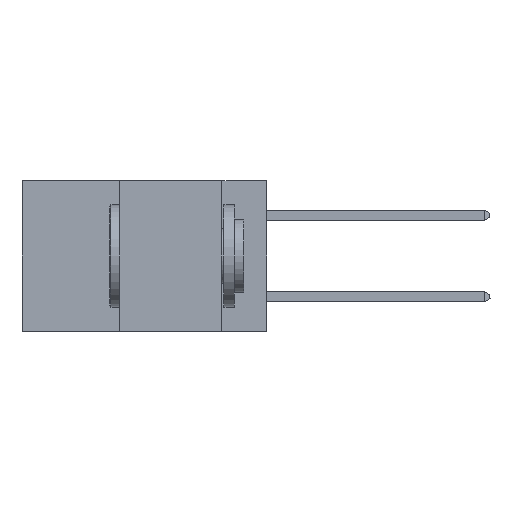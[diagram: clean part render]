
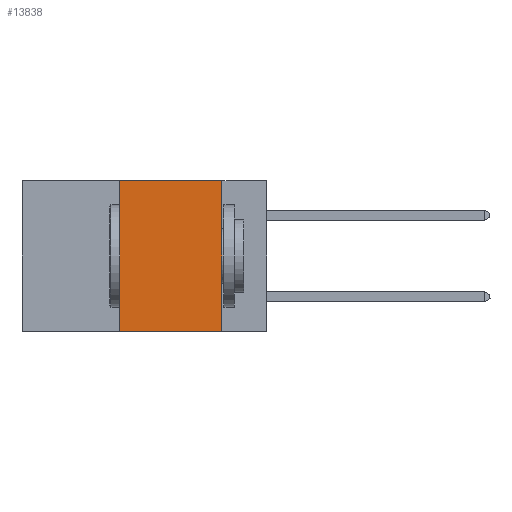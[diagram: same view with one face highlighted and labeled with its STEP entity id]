
A CAD part, left-side view. The second image highlights one B-rep face of the part: STEP entity #13838.
In plain terms, the highlighted planar face has unit normal (-1, 0, 0).
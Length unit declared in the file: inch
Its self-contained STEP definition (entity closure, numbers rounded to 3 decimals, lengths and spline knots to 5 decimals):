
#1724 = DIRECTION ( 'NONE',  ( 0., 0., -1. ) ) ;
#2192 = EDGE_CURVE ( 'NONE', #13459, #39753, #39829, .T. ) ;
#2530 = LINE ( 'NONE', #43156, #29284 ) ;
#3048 = VECTOR ( 'NONE', #5302, 39.37008 ) ;
#4427 = FACE_OUTER_BOUND ( 'NONE', #24896, .T. ) ;
#4590 = DIRECTION ( 'NONE',  ( 0., 0., -1. ) ) ;
#5158 = CARTESIAN_POINT ( 'NONE',  ( 0., 0.6, 0. ) ) ;
#5302 = DIRECTION ( 'NONE',  ( 0., -1., 0. ) ) ;
#6450 = LINE ( 'NONE', #16934, #42121 ) ;
#6618 = EDGE_CURVE ( 'NONE', #26144, #39753, #2530, .T. ) ;
#9150 = CARTESIAN_POINT ( 'NONE',  ( 0., 0.11, -0.37 ) ) ;
#10338 = CARTESIAN_POINT ( 'NONE',  ( 0., 0.11, 0. ) ) ;
#12440 = LINE ( 'NONE', #5158, #3048 ) ;
#13459 = VERTEX_POINT ( 'NONE', #44011 ) ;
#13483 = VECTOR ( 'NONE', #20515, 39.37008 ) ;
#13838 = ADVANCED_FACE ( 'NONE', ( #4427 ), #18582, .F. ) ;
#16684 = ORIENTED_EDGE ( 'NONE', *, *, #6618, .F. ) ;
#16934 = CARTESIAN_POINT ( 'NONE',  ( 0., 0.36, 0. ) ) ;
#18582 = PLANE ( 'NONE',  #23980 ) ;
#18618 = VERTEX_POINT ( 'NONE', #26687 ) ;
#18862 = ORIENTED_EDGE ( 'NONE', *, *, #42453, .F. ) ;
#20515 = DIRECTION ( 'NONE',  ( 0., -1., 0. ) ) ;
#21028 = ORIENTED_EDGE ( 'NONE', *, *, #2192, .T. ) ;
#22050 = CARTESIAN_POINT ( 'NONE',  ( 0., 0.6, 0. ) ) ;
#23980 = AXIS2_PLACEMENT_3D ( 'NONE', #22050, #25537, #4590 ) ;
#24896 = EDGE_LOOP ( 'NONE', ( #16684, #36003, #18862, #21028 ) ) ;
#25537 = DIRECTION ( 'NONE',  ( 1., 0., 0. ) ) ;
#26144 = VERTEX_POINT ( 'NONE', #10338 ) ;
#26687 = CARTESIAN_POINT ( 'NONE',  ( 0., 0.36, 0. ) ) ;
#29284 = VECTOR ( 'NONE', #1724, 39.37008 ) ;
#35425 = EDGE_CURVE ( 'NONE', #18618, #26144, #12440, .T. ) ;
#36003 = ORIENTED_EDGE ( 'NONE', *, *, #35425, .F. ) ;
#37465 = DIRECTION ( 'NONE',  ( 0., 0., 1. ) ) ;
#39753 = VERTEX_POINT ( 'NONE', #9150 ) ;
#39829 = LINE ( 'NONE', #44379, #13483 ) ;
#42121 = VECTOR ( 'NONE', #37465, 39.37008 ) ;
#42453 = EDGE_CURVE ( 'NONE', #13459, #18618, #6450, .T. ) ;
#43156 = CARTESIAN_POINT ( 'NONE',  ( 0., 0.11, 0. ) ) ;
#44011 = CARTESIAN_POINT ( 'NONE',  ( 0., 0.36, -0.37 ) ) ;
#44379 = CARTESIAN_POINT ( 'NONE',  ( 0., 0.6, -0.37 ) ) ;
